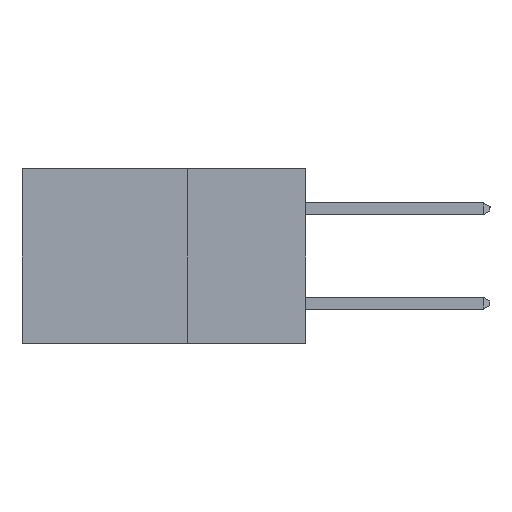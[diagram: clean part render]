
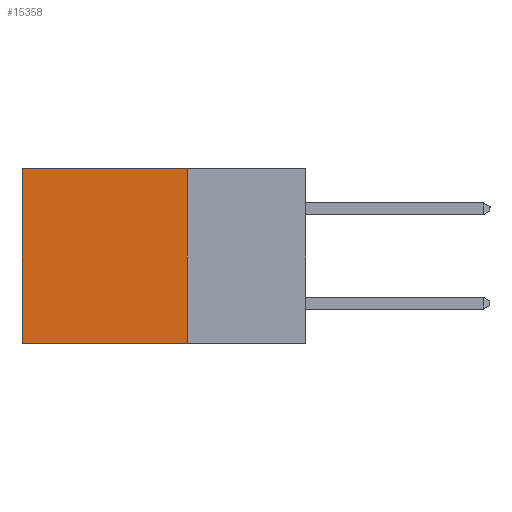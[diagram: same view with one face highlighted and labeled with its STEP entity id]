
A CAD part, left-side view. The second image highlights one B-rep face of the part: STEP entity #15358.
In plain terms, the highlighted planar face has unit normal (-1, 0, 0).
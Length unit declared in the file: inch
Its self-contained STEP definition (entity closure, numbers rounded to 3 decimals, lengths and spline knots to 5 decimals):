
#92 = EDGE_CURVE ( 'NONE', #15715, #10467, #7375, .T. ) ;
#558 = VECTOR ( 'NONE', #11047, 39.37008 ) ;
#1311 = CARTESIAN_POINT ( 'NONE',  ( 0.2615, 0.25, -0.37 ) ) ;
#1799 = VECTOR ( 'NONE', #11005, 39.37008 ) ;
#2004 = CARTESIAN_POINT ( 'NONE',  ( 0.2615, 0.6, -0.37 ) ) ;
#2389 = ORIENTED_EDGE ( 'NONE', *, *, #13102, .F. ) ;
#2472 = CARTESIAN_POINT ( 'NONE',  ( 0.2615, 0.25, -0.37 ) ) ;
#2671 = CARTESIAN_POINT ( 'NONE',  ( 0.2615, 0.25, -0.37 ) ) ;
#3419 = DIRECTION ( 'NONE',  ( 1., 0., 0. ) ) ;
#4200 = CARTESIAN_POINT ( 'NONE',  ( 0.2615, 0.25, 0. ) ) ;
#4212 = VECTOR ( 'NONE', #11097, 39.37008 ) ;
#5472 = CARTESIAN_POINT ( 'NONE',  ( 0.2615, 0.25, -0.37 ) ) ;
#5666 = VERTEX_POINT ( 'NONE', #5472 ) ;
#6237 = CARTESIAN_POINT ( 'NONE',  ( 0.2615, 0.25, 0. ) ) ;
#7346 = DIRECTION ( 'NONE',  ( 0., 0., -1. ) ) ;
#7375 = LINE ( 'NONE', #6237, #4212 ) ;
#7737 = ORIENTED_EDGE ( 'NONE', *, *, #9448, .T. ) ;
#8475 = PLANE ( 'NONE',  #9624 ) ;
#9151 = CARTESIAN_POINT ( 'NONE',  ( 0.2615, 0.6, 0. ) ) ;
#9448 = EDGE_CURVE ( 'NONE', #10467, #9645, #12845, .T. ) ;
#9624 = AXIS2_PLACEMENT_3D ( 'NONE', #2472, #3419, #7346 ) ;
#9645 = VERTEX_POINT ( 'NONE', #2004 ) ;
#9873 = LINE ( 'NONE', #2671, #1799 ) ;
#10224 = CARTESIAN_POINT ( 'NONE',  ( 0.2615, 0.6, -0.37 ) ) ;
#10467 = VERTEX_POINT ( 'NONE', #9151 ) ;
#10971 = VECTOR ( 'NONE', #13811, 39.37008 ) ;
#11005 = DIRECTION ( 'NONE',  ( 0., 1., 0. ) ) ;
#11047 = DIRECTION ( 'NONE',  ( 0., 0., -1. ) ) ;
#11097 = DIRECTION ( 'NONE',  ( 0., 1., 0. ) ) ;
#12083 = EDGE_CURVE ( 'NONE', #5666, #9645, #9873, .T. ) ;
#12109 = FACE_OUTER_BOUND ( 'NONE', #13265, .T. ) ;
#12246 = LINE ( 'NONE', #1311, #558 ) ;
#12845 = LINE ( 'NONE', #10224, #10971 ) ;
#13102 = EDGE_CURVE ( 'NONE', #15715, #5666, #12246, .T. ) ;
#13265 = EDGE_LOOP ( 'NONE', ( #7737, #15660, #2389, #14916 ) ) ;
#13811 = DIRECTION ( 'NONE',  ( 0., 0., -1. ) ) ;
#14916 = ORIENTED_EDGE ( 'NONE', *, *, #92, .T. ) ;
#15358 = ADVANCED_FACE ( 'NONE', ( #12109 ), #8475, .F. ) ;
#15660 = ORIENTED_EDGE ( 'NONE', *, *, #12083, .F. ) ;
#15715 = VERTEX_POINT ( 'NONE', #4200 ) ;
